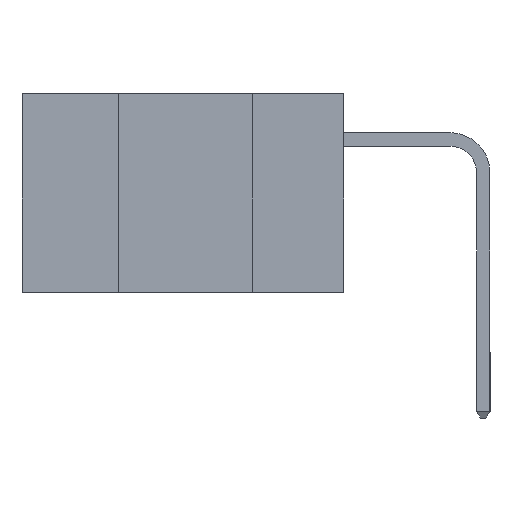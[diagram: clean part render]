
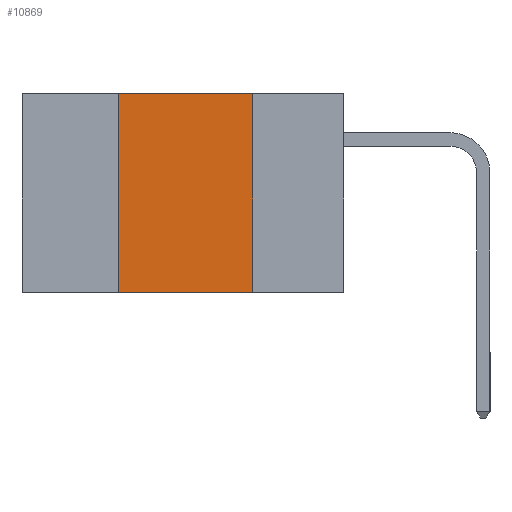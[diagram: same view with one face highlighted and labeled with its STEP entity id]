
A CAD part, left-side view. The second image highlights one B-rep face of the part: STEP entity #10869.
In plain terms, the highlighted planar face has unit normal (-1, 0, 0).
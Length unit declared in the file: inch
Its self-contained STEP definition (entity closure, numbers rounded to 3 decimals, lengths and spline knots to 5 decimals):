
#746 = EDGE_CURVE ( 'NONE', #7849, #6308, #7355, .T. ) ;
#1573 = EDGE_CURVE ( 'NONE', #2784, #7849, #10511, .T. ) ;
#1647 = DIRECTION ( 'NONE',  ( 0., -1., 0. ) ) ;
#1652 = CARTESIAN_POINT ( 'NONE',  ( 0., 0.42, 0. ) ) ;
#1979 = ORIENTED_EDGE ( 'NONE', *, *, #1573, .F. ) ;
#2100 = CARTESIAN_POINT ( 'NONE',  ( 0., 0.42, -0.37 ) ) ;
#2607 = AXIS2_PLACEMENT_3D ( 'NONE', #2840, #10400, #5943 ) ;
#2764 = VECTOR ( 'NONE', #9471, 39.37008 ) ;
#2784 = VERTEX_POINT ( 'NONE', #2100 ) ;
#2840 = CARTESIAN_POINT ( 'NONE',  ( 0., 0.6, 0. ) ) ;
#3081 = CARTESIAN_POINT ( 'NONE',  ( 0., 0.42, -0.37 ) ) ;
#3612 = VECTOR ( 'NONE', #9417, 39.37008 ) ;
#3793 = VERTEX_POINT ( 'NONE', #8859 ) ;
#4770 = EDGE_LOOP ( 'NONE', ( #13831, #13118, #1979, #13796 ) ) ;
#5943 = DIRECTION ( 'NONE',  ( 0., 0., -1. ) ) ;
#6032 = EDGE_CURVE ( 'NONE', #6308, #3793, #12755, .T. ) ;
#6308 = VERTEX_POINT ( 'NONE', #9143 ) ;
#6323 = DIRECTION ( 'NONE',  ( 0., 0., 1. ) ) ;
#6337 = EDGE_CURVE ( 'NONE', #2784, #3793, #8330, .T. ) ;
#7163 = VECTOR ( 'NONE', #6323, 39.37008 ) ;
#7219 = CARTESIAN_POINT ( 'NONE',  ( 0., 0.6, -0.37 ) ) ;
#7355 = LINE ( 'NONE', #10538, #2764 ) ;
#7849 = VERTEX_POINT ( 'NONE', #1652 ) ;
#8184 = FACE_OUTER_BOUND ( 'NONE', #4770, .T. ) ;
#8330 = LINE ( 'NONE', #7219, #12563 ) ;
#8859 = CARTESIAN_POINT ( 'NONE',  ( 0., 0.17, -0.37 ) ) ;
#9143 = CARTESIAN_POINT ( 'NONE',  ( 0., 0.17, 0. ) ) ;
#9417 = DIRECTION ( 'NONE',  ( 0., 0., -1. ) ) ;
#9471 = DIRECTION ( 'NONE',  ( 0., -1., 0. ) ) ;
#10400 = DIRECTION ( 'NONE',  ( 1., 0., 0. ) ) ;
#10511 = LINE ( 'NONE', #3081, #7163 ) ;
#10538 = CARTESIAN_POINT ( 'NONE',  ( 0., 0.6, 0. ) ) ;
#10869 = ADVANCED_FACE ( 'NONE', ( #8184 ), #11237, .F. ) ;
#11237 = PLANE ( 'NONE',  #2607 ) ;
#11884 = CARTESIAN_POINT ( 'NONE',  ( 0., 0.17, -0.37 ) ) ;
#12563 = VECTOR ( 'NONE', #1647, 39.37008 ) ;
#12755 = LINE ( 'NONE', #11884, #3612 ) ;
#13118 = ORIENTED_EDGE ( 'NONE', *, *, #746, .F. ) ;
#13796 = ORIENTED_EDGE ( 'NONE', *, *, #6337, .T. ) ;
#13831 = ORIENTED_EDGE ( 'NONE', *, *, #6032, .F. ) ;
